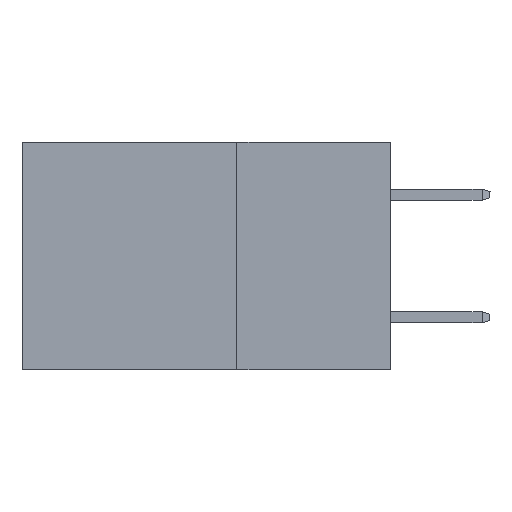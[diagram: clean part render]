
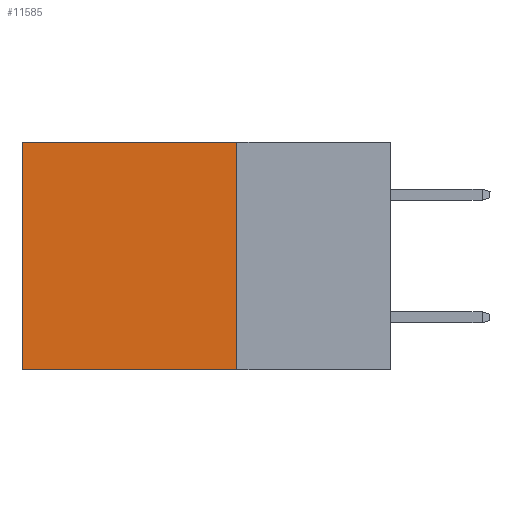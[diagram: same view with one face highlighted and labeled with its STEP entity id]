
A CAD part, left-side view. The second image highlights one B-rep face of the part: STEP entity #11585.
In plain terms, the highlighted planar face has unit normal (-1, 0, 0).
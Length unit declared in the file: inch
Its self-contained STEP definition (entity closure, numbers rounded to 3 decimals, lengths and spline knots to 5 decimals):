
#699 = VERTEX_POINT ( 'NONE', #4402 ) ;
#1865 = VERTEX_POINT ( 'NONE', #11599 ) ;
#2570 = CARTESIAN_POINT ( 'NONE',  ( 0.2875, 0.6, 0. ) ) ;
#2585 = VECTOR ( 'NONE', #11729, 39.37008 ) ;
#3459 = DIRECTION ( 'NONE',  ( 0., 0., -1. ) ) ;
#3893 = LINE ( 'NONE', #7186, #14289 ) ;
#3950 = ORIENTED_EDGE ( 'NONE', *, *, #14004, .F. ) ;
#4402 = CARTESIAN_POINT ( 'NONE',  ( 0.2875, 0.25, -0.37 ) ) ;
#5004 = EDGE_LOOP ( 'NONE', ( #12016, #3950, #11807, #17326 ) ) ;
#6360 = FACE_OUTER_BOUND ( 'NONE', #5004, .T. ) ;
#7186 = CARTESIAN_POINT ( 'NONE',  ( 0.2875, 0.25, -0.37 ) ) ;
#7192 = LINE ( 'NONE', #19409, #2585 ) ;
#7392 = VECTOR ( 'NONE', #3459, 39.37008 ) ;
#8753 = DIRECTION ( 'NONE',  ( 1., 0., 0. ) ) ;
#8805 = VECTOR ( 'NONE', #9602, 39.37008 ) ;
#9091 = VERTEX_POINT ( 'NONE', #11824 ) ;
#9602 = DIRECTION ( 'NONE',  ( 0., 0., -1. ) ) ;
#9744 = EDGE_CURVE ( 'NONE', #1865, #11603, #7192, .T. ) ;
#11211 = CARTESIAN_POINT ( 'NONE',  ( 0.2875, 0.25, 0. ) ) ;
#11585 = ADVANCED_FACE ( 'NONE', ( #6360 ), #14869, .F. ) ;
#11599 = CARTESIAN_POINT ( 'NONE',  ( 0.2875, 0.25, 0. ) ) ;
#11603 = VERTEX_POINT ( 'NONE', #2570 ) ;
#11729 = DIRECTION ( 'NONE',  ( 0., 1., 0. ) ) ;
#11807 = ORIENTED_EDGE ( 'NONE', *, *, #19074, .F. ) ;
#11824 = CARTESIAN_POINT ( 'NONE',  ( 0.2875, 0.6, -0.37 ) ) ;
#12016 = ORIENTED_EDGE ( 'NONE', *, *, #12690, .T. ) ;
#12424 = LINE ( 'NONE', #15693, #8805 ) ;
#12690 = EDGE_CURVE ( 'NONE', #11603, #9091, #12424, .T. ) ;
#14004 = EDGE_CURVE ( 'NONE', #699, #9091, #3893, .T. ) ;
#14289 = VECTOR ( 'NONE', #19557, 39.37008 ) ;
#14869 = PLANE ( 'NONE',  #16910 ) ;
#15693 = CARTESIAN_POINT ( 'NONE',  ( 0.2875, 0.6, 0. ) ) ;
#16910 = AXIS2_PLACEMENT_3D ( 'NONE', #18025, #8753, #19546 ) ;
#17326 = ORIENTED_EDGE ( 'NONE', *, *, #9744, .T. ) ;
#18025 = CARTESIAN_POINT ( 'NONE',  ( 0.2875, 0.25, 0. ) ) ;
#19074 = EDGE_CURVE ( 'NONE', #1865, #699, #19748, .T. ) ;
#19409 = CARTESIAN_POINT ( 'NONE',  ( 0.2875, 0.25, 0. ) ) ;
#19546 = DIRECTION ( 'NONE',  ( 0., 0., -1. ) ) ;
#19557 = DIRECTION ( 'NONE',  ( 0., 1., 0. ) ) ;
#19748 = LINE ( 'NONE', #11211, #7392 ) ;
